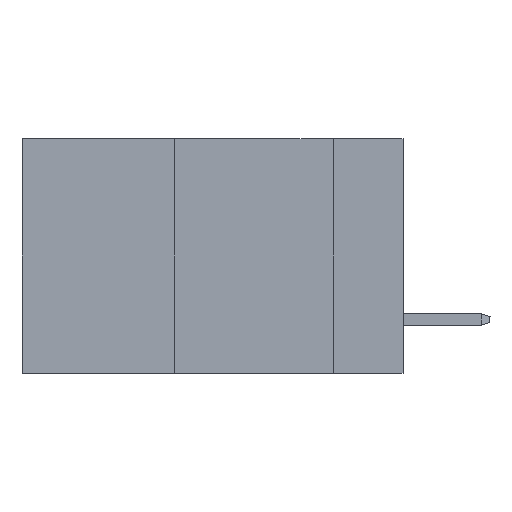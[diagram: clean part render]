
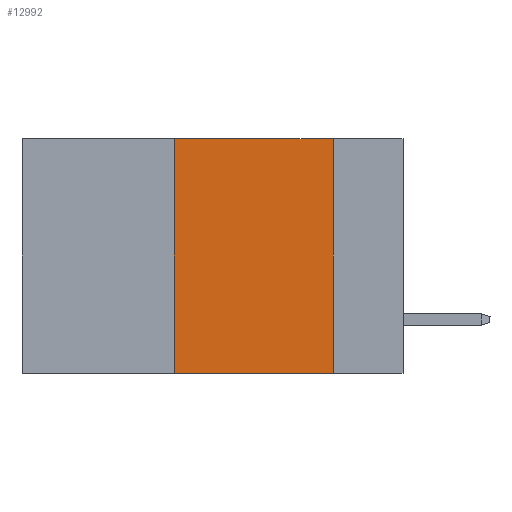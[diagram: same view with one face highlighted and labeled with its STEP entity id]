
A CAD part, left-side view. The second image highlights one B-rep face of the part: STEP entity #12992.
In plain terms, the highlighted planar face has unit normal (-1, 0, 0).
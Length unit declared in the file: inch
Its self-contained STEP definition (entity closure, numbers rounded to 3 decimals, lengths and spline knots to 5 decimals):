
#98 = ORIENTED_EDGE ( 'NONE', *, *, #15485, .F. ) ;
#1536 = LINE ( 'NONE', #10553, #5700 ) ;
#2794 = FACE_OUTER_BOUND ( 'NONE', #12390, .T. ) ;
#2822 = DIRECTION ( 'NONE',  ( 0., -1., 0. ) ) ;
#3168 = ORIENTED_EDGE ( 'NONE', *, *, #18422, .F. ) ;
#3196 = VECTOR ( 'NONE', #22490, 39.37008 ) ;
#3442 = CARTESIAN_POINT ( 'NONE',  ( 0., 0.36, -0.37 ) ) ;
#3929 = VERTEX_POINT ( 'NONE', #12668 ) ;
#4631 = LINE ( 'NONE', #12013, #6287 ) ;
#4846 = DIRECTION ( 'NONE',  ( 1., 0., 0. ) ) ;
#5055 = VERTEX_POINT ( 'NONE', #11272 ) ;
#5311 = AXIS2_PLACEMENT_3D ( 'NONE', #23164, #4846, #10125 ) ;
#5700 = VECTOR ( 'NONE', #23460, 39.37008 ) ;
#6082 = CARTESIAN_POINT ( 'NONE',  ( 0., 0.11, 0. ) ) ;
#6287 = VECTOR ( 'NONE', #2822, 39.37008 ) ;
#6290 = PLANE ( 'NONE',  #5311 ) ;
#7401 = CARTESIAN_POINT ( 'NONE',  ( 0., 0.36, 0. ) ) ;
#8432 = VERTEX_POINT ( 'NONE', #3442 ) ;
#9051 = VECTOR ( 'NONE', #16924, 39.37008 ) ;
#10125 = DIRECTION ( 'NONE',  ( 0., 0., -1. ) ) ;
#10553 = CARTESIAN_POINT ( 'NONE',  ( 0., 0.6, -0.37 ) ) ;
#10624 = ORIENTED_EDGE ( 'NONE', *, *, #22286, .T. ) ;
#11272 = CARTESIAN_POINT ( 'NONE',  ( 0., 0.11, 0. ) ) ;
#12013 = CARTESIAN_POINT ( 'NONE',  ( 0., 0.6, 0. ) ) ;
#12390 = EDGE_LOOP ( 'NONE', ( #98, #19877, #3168, #10624 ) ) ;
#12668 = CARTESIAN_POINT ( 'NONE',  ( 0., 0.11, -0.37 ) ) ;
#12992 = ADVANCED_FACE ( 'NONE', ( #2794 ), #6290, .F. ) ;
#13100 = LINE ( 'NONE', #7401, #9051 ) ;
#13355 = LINE ( 'NONE', #6082, #3196 ) ;
#14350 = VERTEX_POINT ( 'NONE', #17379 ) ;
#15485 = EDGE_CURVE ( 'NONE', #5055, #3929, #13355, .T. ) ;
#16800 = EDGE_CURVE ( 'NONE', #14350, #5055, #4631, .T. ) ;
#16924 = DIRECTION ( 'NONE',  ( 0., 0., 1. ) ) ;
#17379 = CARTESIAN_POINT ( 'NONE',  ( 0., 0.36, 0. ) ) ;
#18422 = EDGE_CURVE ( 'NONE', #8432, #14350, #13100, .T. ) ;
#19877 = ORIENTED_EDGE ( 'NONE', *, *, #16800, .F. ) ;
#22286 = EDGE_CURVE ( 'NONE', #8432, #3929, #1536, .T. ) ;
#22490 = DIRECTION ( 'NONE',  ( 0., 0., -1. ) ) ;
#23164 = CARTESIAN_POINT ( 'NONE',  ( 0., 0.6, 0. ) ) ;
#23460 = DIRECTION ( 'NONE',  ( 0., -1., 0. ) ) ;
